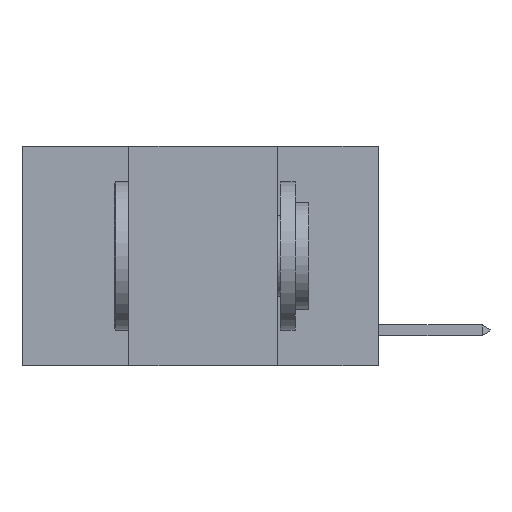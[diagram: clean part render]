
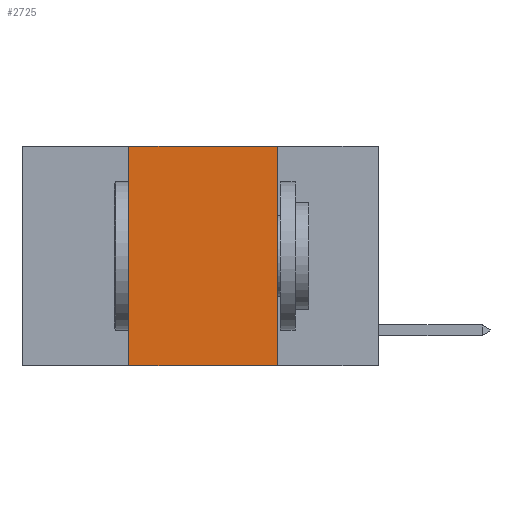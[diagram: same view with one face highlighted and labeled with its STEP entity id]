
A CAD part, left-side view. The second image highlights one B-rep face of the part: STEP entity #2725.
In plain terms, the highlighted planar face has unit normal (-1, 0, 0).
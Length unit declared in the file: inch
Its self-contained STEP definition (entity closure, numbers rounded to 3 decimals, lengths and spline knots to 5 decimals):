
#2387 = CARTESIAN_POINT ( 'NONE',  ( 0., 0.42, 0. ) ) ;
#2725 = ADVANCED_FACE ( 'NONE', ( #8467 ), #5313, .F. ) ;
#2953 = DIRECTION ( 'NONE',  ( 0., 0., -1. ) ) ;
#3094 = VERTEX_POINT ( 'NONE', #18618 ) ;
#3603 = CARTESIAN_POINT ( 'NONE',  ( 0., 0.6, -0.37 ) ) ;
#3629 = VERTEX_POINT ( 'NONE', #12385 ) ;
#4984 = VECTOR ( 'NONE', #2953, 39.37008 ) ;
#5026 = EDGE_CURVE ( 'NONE', #14693, #3629, #14717, .T. ) ;
#5044 = DIRECTION ( 'NONE',  ( 0., 0., -1. ) ) ;
#5071 = DIRECTION ( 'NONE',  ( 1., 0., 0. ) ) ;
#5076 = DIRECTION ( 'NONE',  ( 0., -1., 0. ) ) ;
#5095 = CARTESIAN_POINT ( 'NONE',  ( 0., 0.6, 0. ) ) ;
#5313 = PLANE ( 'NONE',  #8511 ) ;
#5336 = VECTOR ( 'NONE', #5076, 39.37008 ) ;
#6224 = ORIENTED_EDGE ( 'NONE', *, *, #10631, .F. ) ;
#6275 = LINE ( 'NONE', #3603, #5336 ) ;
#6950 = CARTESIAN_POINT ( 'NONE',  ( 0., 0.17, 0. ) ) ;
#7159 = EDGE_LOOP ( 'NONE', ( #6224, #9281, #14062, #15927 ) ) ;
#7270 = VECTOR ( 'NONE', #18681, 39.37008 ) ;
#8467 = FACE_OUTER_BOUND ( 'NONE', #7159, .T. ) ;
#8511 = AXIS2_PLACEMENT_3D ( 'NONE', #5095, #5071, #5044 ) ;
#9281 = ORIENTED_EDGE ( 'NONE', *, *, #16505, .F. ) ;
#10158 = VECTOR ( 'NONE', #11404, 39.37008 ) ;
#10631 = EDGE_CURVE ( 'NONE', #11985, #3094, #12879, .T. ) ;
#11404 = DIRECTION ( 'NONE',  ( 0., -1., 0. ) ) ;
#11985 = VERTEX_POINT ( 'NONE', #6950 ) ;
#12385 = CARTESIAN_POINT ( 'NONE',  ( 0., 0.42, 0. ) ) ;
#12879 = LINE ( 'NONE', #13313, #4984 ) ;
#13313 = CARTESIAN_POINT ( 'NONE',  ( 0., 0.17, 0. ) ) ;
#14062 = ORIENTED_EDGE ( 'NONE', *, *, #5026, .F. ) ;
#14402 = EDGE_CURVE ( 'NONE', #14693, #3094, #6275, .T. ) ;
#14693 = VERTEX_POINT ( 'NONE', #17601 ) ;
#14717 = LINE ( 'NONE', #2387, #7270 ) ;
#15927 = ORIENTED_EDGE ( 'NONE', *, *, #14402, .T. ) ;
#15966 = CARTESIAN_POINT ( 'NONE',  ( 0., 0.6, 0. ) ) ;
#16505 = EDGE_CURVE ( 'NONE', #3629, #11985, #17655, .T. ) ;
#17601 = CARTESIAN_POINT ( 'NONE',  ( 0., 0.42, -0.37 ) ) ;
#17655 = LINE ( 'NONE', #15966, #10158 ) ;
#18618 = CARTESIAN_POINT ( 'NONE',  ( 0., 0.17, -0.37 ) ) ;
#18681 = DIRECTION ( 'NONE',  ( 0., 0., 1. ) ) ;
